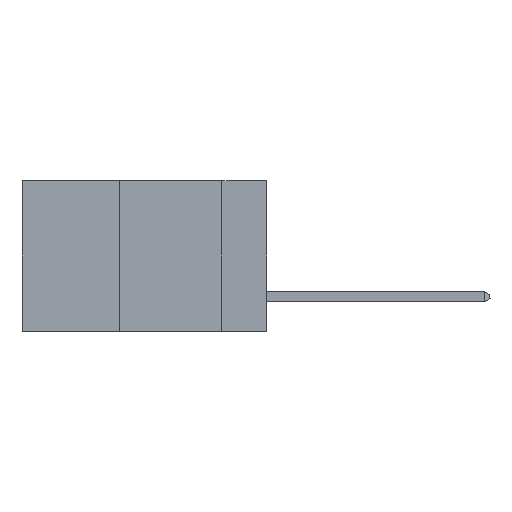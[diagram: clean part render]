
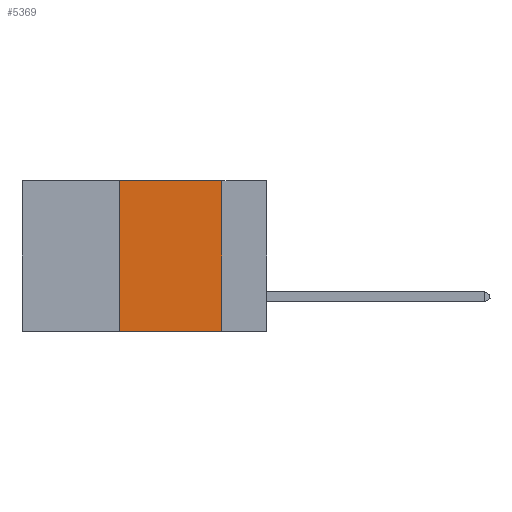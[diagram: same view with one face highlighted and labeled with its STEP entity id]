
A CAD part, left-side view. The second image highlights one B-rep face of the part: STEP entity #5369.
In plain terms, the highlighted planar face has unit normal (-1, 0, 0).
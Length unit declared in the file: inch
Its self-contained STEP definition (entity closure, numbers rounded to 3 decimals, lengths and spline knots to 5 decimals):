
#972 = ORIENTED_EDGE ( 'NONE', *, *, #1737, .T. ) ;
#1296 = EDGE_CURVE ( 'NONE', #13215, #1846, #13814, .T. ) ;
#1737 = EDGE_CURVE ( 'NONE', #8177, #16044, #15183, .T. ) ;
#1846 = VERTEX_POINT ( 'NONE', #9684 ) ;
#2542 = DIRECTION ( 'NONE',  ( 0., 0., -1. ) ) ;
#3112 = CARTESIAN_POINT ( 'NONE',  ( 0., 0.6, 0. ) ) ;
#3411 = VECTOR ( 'NONE', #11087, 39.37008 ) ;
#4452 = DIRECTION ( 'NONE',  ( 1., 0., 0. ) ) ;
#4600 = DIRECTION ( 'NONE',  ( 0., 0., 1. ) ) ;
#4675 = DIRECTION ( 'NONE',  ( 0., -1., 0. ) ) ;
#4908 = CARTESIAN_POINT ( 'NONE',  ( 0., 0.11, 0. ) ) ;
#5369 = ADVANCED_FACE ( 'NONE', ( #16962 ), #16700, .F. ) ;
#6774 = ORIENTED_EDGE ( 'NONE', *, *, #6801, .F. ) ;
#6801 = EDGE_CURVE ( 'NONE', #1846, #16044, #14248, .T. ) ;
#7998 = ORIENTED_EDGE ( 'NONE', *, *, #8054, .F. ) ;
#8054 = EDGE_CURVE ( 'NONE', #8177, #13215, #15221, .T. ) ;
#8120 = EDGE_LOOP ( 'NONE', ( #6774, #13019, #7998, #972 ) ) ;
#8177 = VERTEX_POINT ( 'NONE', #15842 ) ;
#8480 = VECTOR ( 'NONE', #4600, 39.37008 ) ;
#9684 = CARTESIAN_POINT ( 'NONE',  ( 0., 0.11, 0. ) ) ;
#11087 = DIRECTION ( 'NONE',  ( 0., 0., -1. ) ) ;
#12843 = VECTOR ( 'NONE', #4675, 39.37008 ) ;
#13019 = ORIENTED_EDGE ( 'NONE', *, *, #1296, .F. ) ;
#13215 = VERTEX_POINT ( 'NONE', #16745 ) ;
#13543 = CARTESIAN_POINT ( 'NONE',  ( 0., 0.11, -0.37 ) ) ;
#13675 = CARTESIAN_POINT ( 'NONE',  ( 0., 0.6, 0. ) ) ;
#13814 = LINE ( 'NONE', #3112, #12843 ) ;
#13831 = CARTESIAN_POINT ( 'NONE',  ( 0., 0.36, 0. ) ) ;
#14248 = LINE ( 'NONE', #4908, #3411 ) ;
#15183 = LINE ( 'NONE', #15745, #18798 ) ;
#15221 = LINE ( 'NONE', #13831, #8480 ) ;
#15745 = CARTESIAN_POINT ( 'NONE',  ( 0., 0.6, -0.37 ) ) ;
#15842 = CARTESIAN_POINT ( 'NONE',  ( 0., 0.36, -0.37 ) ) ;
#16044 = VERTEX_POINT ( 'NONE', #13543 ) ;
#16700 = PLANE ( 'NONE',  #18351 ) ;
#16745 = CARTESIAN_POINT ( 'NONE',  ( 0., 0.36, 0. ) ) ;
#16962 = FACE_OUTER_BOUND ( 'NONE', #8120, .T. ) ;
#18351 = AXIS2_PLACEMENT_3D ( 'NONE', #13675, #4452, #2542 ) ;
#18772 = DIRECTION ( 'NONE',  ( 0., -1., 0. ) ) ;
#18798 = VECTOR ( 'NONE', #18772, 39.37008 ) ;
